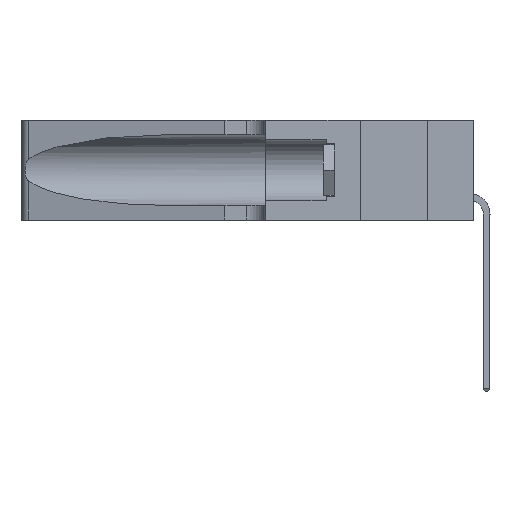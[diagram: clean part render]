
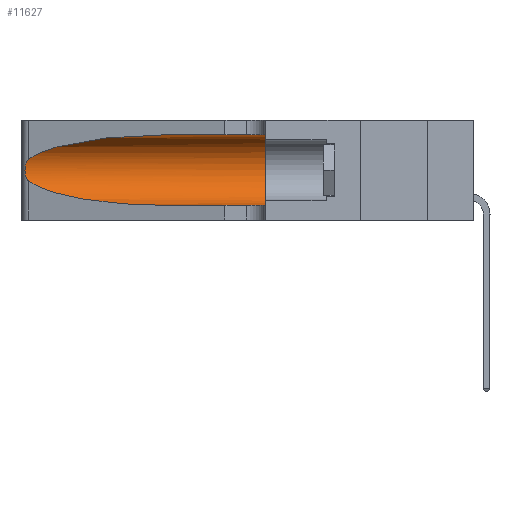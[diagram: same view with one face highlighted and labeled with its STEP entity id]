
A CAD part, left-side view. The second image highlights one B-rep face of the part: STEP entity #11627.
In plain terms, the highlighted cylindrical face has radius 3.308 mm (diameter 6.617 mm), a partial arc.
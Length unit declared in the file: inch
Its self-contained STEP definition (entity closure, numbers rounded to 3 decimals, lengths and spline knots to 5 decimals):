
#314 = CARTESIAN_POINT ( 'NONE',  ( 0.25487, 1.22718, 0.22369 ) ) ;
#379 = CARTESIAN_POINT ( 'NONE',  ( 0.2373, 1.15595, 0.28018 ) ) ;
#416 = AXIS2_PLACEMENT_3D ( 'NONE', #8786, #2558, #16764 ) ;
#1565 = CARTESIAN_POINT ( 'NONE',  ( 0.1305, 0.35, 0.05475 ) ) ;
#2175 = CARTESIAN_POINT ( 'NONE',  ( 0.1305, 0.72297, 0.05475 ) ) ;
#2558 = DIRECTION ( 'NONE',  ( 0., 1., 0. ) ) ;
#2781 = CARTESIAN_POINT ( 'NONE',  ( 0.25487, 1.22718, 0.14631 ) ) ;
#3343 = ORIENTED_EDGE ( 'NONE', *, *, #23437, .T. ) ;
#3365 = EDGE_CURVE ( 'NONE', #14951, #21096, #21630, .T. ) ;
#3525 = CARTESIAN_POINT ( 'NONE',  ( 0.25854, 1.2359, 0.20912 ) ) ;
#5489 = CARTESIAN_POINT ( 'NONE',  ( 0.1305, 0.72297, 0.31525 ) ) ;
#5575 = CARTESIAN_POINT ( 'NONE',  ( 0.26075, 1.23896, 0.178 ) ) ;
#5829 = CARTESIAN_POINT ( 'NONE',  ( 0.25639, 1.23186, 0.15144 ) ) ;
#5861 = EDGE_CURVE ( 'NONE', #22358, #21096, #18913, .T. ) ;
#6591 = CARTESIAN_POINT ( 'NONE',  ( 0.1305, 1.61858, 0.31525 ) ) ;
#6867 = AXIS2_PLACEMENT_3D ( 'NONE', #17068, #25730, #9102 ) ;
#7295 = ORIENTED_EDGE ( 'NONE', *, *, #13461, .T. ) ;
#7648 = CARTESIAN_POINT ( 'NONE',  ( 0.25487, 1.22718, 0.14631 ) ) ;
#7736 = CARTESIAN_POINT ( 'NONE',  ( 0.25487, 1.22718, 0.22369 ) ) ;
#8786 = CARTESIAN_POINT ( 'NONE',  ( 0.1305, 0.35, 0.185 ) ) ;
#9102 = DIRECTION ( 'NONE',  ( 0., 0., -1. ) ) ;
#9411 = ORIENTED_EDGE ( 'NONE', *, *, #15834, .T. ) ;
#10763 = CARTESIAN_POINT ( 'NONE',  ( 0.1305, 0.72297, 0.31525 ) ) ;
#10946 = CARTESIAN_POINT ( 'NONE',  ( 0.25487, 1.22718, 0.14631 ) ) ;
#11627 = ADVANCED_FACE ( 'NONE', ( #25902 ), #13497, .F. ) ;
#13051 = CARTESIAN_POINT ( 'NONE',  ( 0.18966, 0.96281, 0.05475 ) ) ;
#13461 = EDGE_CURVE ( 'NONE', #16480, #22022, #16550, .T. ) ;
#13497 = CYLINDRICAL_SURFACE ( 'NONE', #6867, 0.13025 ) ;
#14554 = CARTESIAN_POINT ( 'NONE',  ( 0.2373, 1.15595, 0.08982 ) ) ;
#14706 = ORIENTED_EDGE ( 'NONE', *, *, #17952, .F. ) ;
#14951 = VERTEX_POINT ( 'NONE', #24299 ) ;
#15834 = EDGE_CURVE ( 'NONE', #22022, #19805, #18167, .T. ) ;
#15871 = ORIENTED_EDGE ( 'NONE', *, *, #5861, .F. ) ;
#15930 = ORIENTED_EDGE ( 'NONE', *, *, #3365, .T. ) ;
#16186 = CARTESIAN_POINT ( 'NONE',  ( 0.1305, 0.35, 0.31525 ) ) ;
#16480 = VERTEX_POINT ( 'NONE', #5489 ) ;
#16550 =( BOUNDED_CURVE ( )  B_SPLINE_CURVE ( 3, ( #10763, #18802, #379, #18991 ),
 .UNSPECIFIED., .F., .T. ) 
 B_SPLINE_CURVE_WITH_KNOTS ( ( 4, 4 ),
 ( 1.5708, 2.84003 ),
 .UNSPECIFIED. ) 
 CURVE ( )  GEOMETRIC_REPRESENTATION_ITEM ( )  RATIONAL_B_SPLINE_CURVE ( ( 1., 0.87, 0.87, 1. ) ) 
 REPRESENTATION_ITEM ( '' )  );
#16764 = DIRECTION ( 'NONE',  ( 0., 0., 1. ) ) ;
#17068 = CARTESIAN_POINT ( 'NONE',  ( 0.1305, 1.61858, 0.185 ) ) ;
#17807 = LINE ( 'NONE', #6591, #24465 ) ;
#17918 = CARTESIAN_POINT ( 'NONE',  ( 0.26075, 1.23896, 0.19203 ) ) ;
#17952 = EDGE_CURVE ( 'NONE', #16480, #22358, #17807, .T. ) ;
#18156 = CARTESIAN_POINT ( 'NONE',  ( 0.25856, 1.23593, 0.16098 ) ) ;
#18167 = B_SPLINE_CURVE_WITH_KNOTS ( 'NONE', 3,
 ( #7736, #26083, #26259, #20115, #3525, #21906, #17918, #5575, #22094, #18156, #19951, #5829, #22256, #7648 ),
 .UNSPECIFIED., .F., .F.,
 ( 4, 2, 2, 2, 2, 2, 4 ),
 ( 0., 0.00027, 0.00053, 0.00107, 0.0016, 0.00187, 0.00214 ),
 .UNSPECIFIED. ) ;
#18802 = CARTESIAN_POINT ( 'NONE',  ( 0.18966, 0.96281, 0.31525 ) ) ;
#18913 = CIRCLE ( 'NONE', #416, 0.13025 ) ;
#18991 = CARTESIAN_POINT ( 'NONE',  ( 0.25487, 1.22718, 0.22369 ) ) ;
#19224 = DIRECTION ( 'NONE',  ( 0., -1., 0. ) ) ;
#19805 = VERTEX_POINT ( 'NONE', #2781 ) ;
#19951 = CARTESIAN_POINT ( 'NONE',  ( 0.25789, 1.23486, 0.15765 ) ) ;
#20115 = CARTESIAN_POINT ( 'NONE',  ( 0.25787, 1.23484, 0.2124 ) ) ;
#20940 = DIRECTION ( 'NONE',  ( 0., -1., 0. ) ) ;
#21096 = VERTEX_POINT ( 'NONE', #1565 ) ;
#21630 = LINE ( 'NONE', #25257, #25771 ) ;
#21702 = EDGE_LOOP ( 'NONE', ( #7295, #9411, #3343, #15930, #15871, #14706 ) ) ;
#21906 = CARTESIAN_POINT ( 'NONE',  ( 0.26018, 1.23835, 0.19895 ) ) ;
#22022 = VERTEX_POINT ( 'NONE', #314 ) ;
#22094 = CARTESIAN_POINT ( 'NONE',  ( 0.26017, 1.23833, 0.17102 ) ) ;
#22256 = CARTESIAN_POINT ( 'NONE',  ( 0.25555, 1.22993, 0.14849 ) ) ;
#22358 = VERTEX_POINT ( 'NONE', #16186 ) ;
#23437 = EDGE_CURVE ( 'NONE', #19805, #14951, #24196, .T. ) ;
#24196 =( BOUNDED_CURVE ( )  B_SPLINE_CURVE ( 3, ( #10946, #14554, #13051, #2175 ),
 .UNSPECIFIED., .F., .T. ) 
 B_SPLINE_CURVE_WITH_KNOTS ( ( 4, 4 ),
 ( 3.44316, 4.71239 ),
 .UNSPECIFIED. ) 
 CURVE ( )  GEOMETRIC_REPRESENTATION_ITEM ( )  RATIONAL_B_SPLINE_CURVE ( ( 1., 0.87, 0.87, 1. ) ) 
 REPRESENTATION_ITEM ( '' )  );
#24299 = CARTESIAN_POINT ( 'NONE',  ( 0.1305, 0.72297, 0.05475 ) ) ;
#24465 = VECTOR ( 'NONE', #20940, 39.37008 ) ;
#25257 = CARTESIAN_POINT ( 'NONE',  ( 0.1305, 1.61858, 0.05475 ) ) ;
#25730 = DIRECTION ( 'NONE',  ( 0., -1., 0. ) ) ;
#25771 = VECTOR ( 'NONE', #19224, 39.37008 ) ;
#25902 = FACE_OUTER_BOUND ( 'NONE', #21702, .T. ) ;
#26083 = CARTESIAN_POINT ( 'NONE',  ( 0.25555, 1.22994, 0.2215 ) ) ;
#26259 = CARTESIAN_POINT ( 'NONE',  ( 0.25639, 1.23184, 0.21858 ) ) ;
